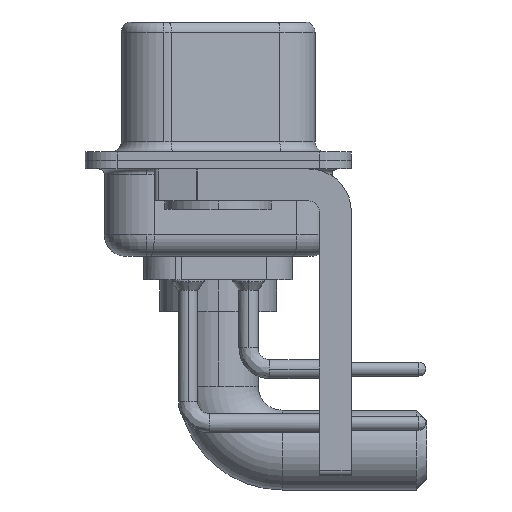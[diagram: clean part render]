
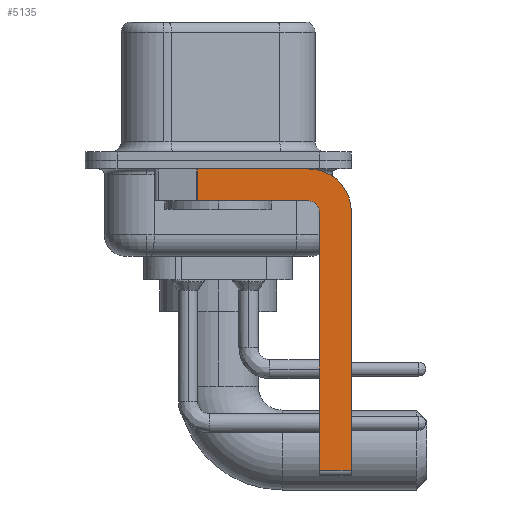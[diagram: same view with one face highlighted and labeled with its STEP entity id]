
A CAD part, left-side view. The second image highlights one B-rep face of the part: STEP entity #5135.
In plain terms, the highlighted planar face has unit normal (-1, 0, 0).
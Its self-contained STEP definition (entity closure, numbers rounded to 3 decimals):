
#94 = EDGE_LOOP ( 'NONE', ( #19733, #12393, #5983, #20560, #14807, #6351, #7625, #3235 ) ) ;
#341 = VECTOR ( 'NONE', #1682, 1000. ) ;
#744 = EDGE_CURVE ( 'NONE', #19781, #9764, #15898, .T. ) ;
#1156 = DIRECTION ( 'NONE',  ( 0., 0., 1. ) ) ;
#1232 = CARTESIAN_POINT ( 'NONE',  ( -2.9, -4.75, -2.4 ) ) ;
#1496 = VERTEX_POINT ( 'NONE', #21345 ) ;
#1682 = DIRECTION ( 'NONE',  ( 0., -1., 0. ) ) ;
#1813 = CARTESIAN_POINT ( 'NONE',  ( -2.9, 3., -0.4 ) ) ;
#1815 = CARTESIAN_POINT ( 'NONE',  ( -2.9, -4.75, -14.55 ) ) ;
#2695 = EDGE_CURVE ( 'NONE', #18354, #1496, #6538, .T. ) ;
#2917 = CARTESIAN_POINT ( 'NONE',  ( -2.9, -4.25, -2.4 ) ) ;
#3235 = ORIENTED_EDGE ( 'NONE', *, *, #10258, .F. ) ;
#3435 = DIRECTION ( 'NONE',  ( 0., 0., 1. ) ) ;
#4931 = DIRECTION ( 'NONE',  ( 0., -1., 0. ) ) ;
#4991 = PLANE ( 'NONE',  #25100 ) ;
#5135 = ADVANCED_FACE ( 'NONE', ( #19685 ), #4991, .F. ) ;
#5737 = CARTESIAN_POINT ( 'NONE',  ( -2.9, -4.75, -14.8 ) ) ;
#5983 = ORIENTED_EDGE ( 'NONE', *, *, #15563, .F. ) ;
#6351 = ORIENTED_EDGE ( 'NONE', *, *, #2695, .T. ) ;
#6538 = LINE ( 'NONE', #15051, #7062 ) ;
#7006 = CARTESIAN_POINT ( 'NONE',  ( -2.9, -4.25, -2.4 ) ) ;
#7062 = VECTOR ( 'NONE', #4931, 1000. ) ;
#7532 = DIRECTION ( 'NONE',  ( 0., 0., -1. ) ) ;
#7625 = ORIENTED_EDGE ( 'NONE', *, *, #10260, .F. ) ;
#7841 = VECTOR ( 'NONE', #3435, 1000. ) ;
#7957 = EDGE_CURVE ( 'NONE', #19781, #22979, #10176, .T. ) ;
#8726 = VECTOR ( 'NONE', #13533, 1000. ) ;
#9077 = CARTESIAN_POINT ( 'NONE',  ( -2.9, -4.25, -1.9 ) ) ;
#9295 = DIRECTION ( 'NONE',  ( 1., 0., 0. ) ) ;
#9478 = CIRCLE ( 'NONE', #19823, 0.5 ) ;
#9764 = VERTEX_POINT ( 'NONE', #25371 ) ;
#10176 = LINE ( 'NONE', #1813, #341 ) ;
#10258 = EDGE_CURVE ( 'NONE', #22979, #18401, #10885, .T. ) ;
#10260 = EDGE_CURVE ( 'NONE', #18401, #1496, #25462, .T. ) ;
#10885 = CIRCLE ( 'NONE', #11724, 2. ) ;
#11724 = AXIS2_PLACEMENT_3D ( 'NONE', #25071, #17399, #13078 ) ;
#12349 = VERTEX_POINT ( 'NONE', #24886 ) ;
#12393 = ORIENTED_EDGE ( 'NONE', *, *, #744, .T. ) ;
#13078 = DIRECTION ( 'NONE',  ( 0., 0., -1. ) ) ;
#13533 = DIRECTION ( 'NONE',  ( 0., 1., 0. ) ) ;
#13603 = DIRECTION ( 'NONE',  ( 0., 0., -1. ) ) ;
#13692 = LINE ( 'NONE', #5737, #7841 ) ;
#13884 = EDGE_CURVE ( 'NONE', #23500, #12349, #9478, .T. ) ;
#14349 = VECTOR ( 'NONE', #15103, 1000. ) ;
#14807 = ORIENTED_EDGE ( 'NONE', *, *, #15317, .F. ) ;
#14914 = CARTESIAN_POINT ( 'NONE',  ( -2.9, 0.978, -0.4 ) ) ;
#15051 = CARTESIAN_POINT ( 'NONE',  ( -2.9, -4.25, -14.55 ) ) ;
#15103 = DIRECTION ( 'NONE',  ( 0., 0., -1. ) ) ;
#15317 = EDGE_CURVE ( 'NONE', #18354, #23500, #13692, .T. ) ;
#15563 = EDGE_CURVE ( 'NONE', #12349, #9764, #25285, .T. ) ;
#15699 = CARTESIAN_POINT ( 'NONE',  ( -2.9, -4.25, -0.4 ) ) ;
#15898 = LINE ( 'NONE', #26407, #16041 ) ;
#16041 = VECTOR ( 'NONE', #7532, 1000. ) ;
#17399 = DIRECTION ( 'NONE',  ( 1., 0., 0. ) ) ;
#18354 = VERTEX_POINT ( 'NONE', #1815 ) ;
#18401 = VERTEX_POINT ( 'NONE', #25943 ) ;
#19685 = FACE_OUTER_BOUND ( 'NONE', #94, .T. ) ;
#19733 = ORIENTED_EDGE ( 'NONE', *, *, #7957, .F. ) ;
#19781 = VERTEX_POINT ( 'NONE', #14914 ) ;
#19823 = AXIS2_PLACEMENT_3D ( 'NONE', #2917, #21649, #1156 ) ;
#20560 = ORIENTED_EDGE ( 'NONE', *, *, #13884, .F. ) ;
#21345 = CARTESIAN_POINT ( 'NONE',  ( -2.9, -6.25, -14.55 ) ) ;
#21649 = DIRECTION ( 'NONE',  ( -1., 0., 0. ) ) ;
#22979 = VERTEX_POINT ( 'NONE', #15699 ) ;
#23500 = VERTEX_POINT ( 'NONE', #1232 ) ;
#24886 = CARTESIAN_POINT ( 'NONE',  ( -2.9, -4.25, -1.9 ) ) ;
#25071 = CARTESIAN_POINT ( 'NONE',  ( -2.9, -4.25, -2.4 ) ) ;
#25100 = AXIS2_PLACEMENT_3D ( 'NONE', #7006, #9295, #13603 ) ;
#25211 = CARTESIAN_POINT ( 'NONE',  ( -2.9, -6.25, -2.4 ) ) ;
#25285 = LINE ( 'NONE', #9077, #8726 ) ;
#25371 = CARTESIAN_POINT ( 'NONE',  ( -2.9, 0.978, -1.9 ) ) ;
#25462 = LINE ( 'NONE', #25211, #14349 ) ;
#25943 = CARTESIAN_POINT ( 'NONE',  ( -2.9, -6.25, -2.4 ) ) ;
#26407 = CARTESIAN_POINT ( 'NONE',  ( -2.9, 0.978, -1.9 ) ) ;
